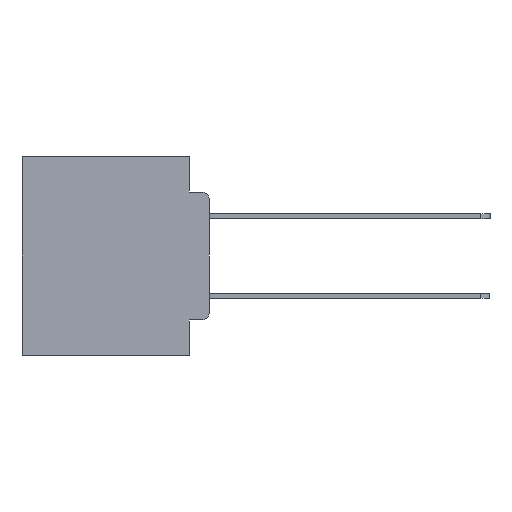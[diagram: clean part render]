
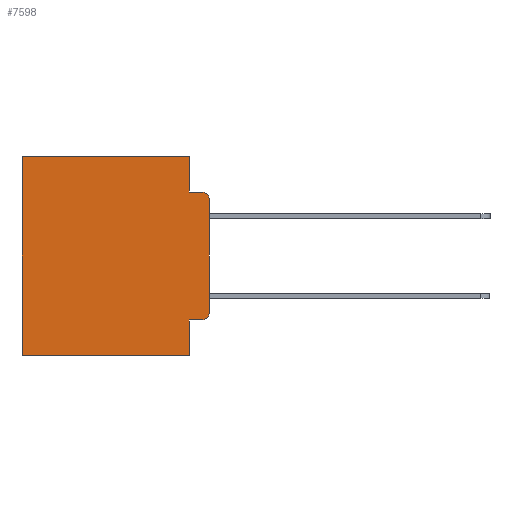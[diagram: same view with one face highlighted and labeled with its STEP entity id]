
A CAD part, left-side view. The second image highlights one B-rep face of the part: STEP entity #7598.
In plain terms, the highlighted planar face has unit normal (-1, 0, 0).
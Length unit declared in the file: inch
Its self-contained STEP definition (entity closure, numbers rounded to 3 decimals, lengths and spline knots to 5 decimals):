
#536 = EDGE_CURVE ( 'NONE', #15988, #26133, #26964, .T. ) ;
#649 = ORIENTED_EDGE ( 'NONE', *, *, #8804, .T. ) ;
#811 = VECTOR ( 'NONE', #26884, 39.37008 ) ;
#1095 = VECTOR ( 'NONE', #17243, 39.37008 ) ;
#1153 = FACE_OUTER_BOUND ( 'NONE', #25852, .T. ) ;
#1531 = CARTESIAN_POINT ( 'NONE',  ( 0.298, 0.473, 0. ) ) ;
#1646 = DIRECTION ( 'NONE',  ( -1., 0., 0. ) ) ;
#1666 = VECTOR ( 'NONE', #23406, 39.37008 ) ;
#1726 = CARTESIAN_POINT ( 'NONE',  ( 0.298, 0.051, -0.0885 ) ) ;
#2433 = EDGE_CURVE ( 'NONE', #15988, #26353, #12940, .T. ) ;
#2542 = ORIENTED_EDGE ( 'NONE', *, *, #2433, .F. ) ;
#2942 = CARTESIAN_POINT ( 'NONE',  ( 0.298, 0.051, -0.4115 ) ) ;
#4128 = CARTESIAN_POINT ( 'NONE',  ( 0.298, 0.02, -0.1085 ) ) ;
#4320 = ORIENTED_EDGE ( 'NONE', *, *, #12339, .F. ) ;
#4534 = ORIENTED_EDGE ( 'NONE', *, *, #19106, .T. ) ;
#4687 = VERTEX_POINT ( 'NONE', #25197 ) ;
#4892 = CARTESIAN_POINT ( 'NONE',  ( 0.298, 0.473, -0.5 ) ) ;
#4972 = ORIENTED_EDGE ( 'NONE', *, *, #25614, .F. ) ;
#5144 = DIRECTION ( 'NONE',  ( 0., -1., 0. ) ) ;
#5269 = AXIS2_PLACEMENT_3D ( 'NONE', #25804, #6248, #22928 ) ;
#5729 = ORIENTED_EDGE ( 'NONE', *, *, #23410, .F. ) ;
#5737 = ORIENTED_EDGE ( 'NONE', *, *, #19331, .T. ) ;
#6018 = AXIS2_PLACEMENT_3D ( 'NONE', #14471, #1646, #16541 ) ;
#6137 = LINE ( 'NONE', #11138, #1666 ) ;
#6248 = DIRECTION ( 'NONE',  ( 1., 0., 0. ) ) ;
#6474 = DIRECTION ( 'NONE',  ( 0., 1., 0. ) ) ;
#6486 = AXIS2_PLACEMENT_3D ( 'NONE', #4128, #9672, #23603 ) ;
#6606 = ORIENTED_EDGE ( 'NONE', *, *, #16039, .T. ) ;
#7159 = ORIENTED_EDGE ( 'NONE', *, *, #14793, .F. ) ;
#7250 = LINE ( 'NONE', #11858, #17108 ) ;
#7393 = LINE ( 'NONE', #1726, #12377 ) ;
#7552 = CARTESIAN_POINT ( 'NONE',  ( 0.298, 0.051, -0.0885 ) ) ;
#7598 = ADVANCED_FACE ( 'NONE', ( #1153 ), #25890, .F. ) ;
#8273 = DIRECTION ( 'NONE',  ( 0., -1., 0. ) ) ;
#8526 = CARTESIAN_POINT ( 'NONE',  ( 0.298, 0., -0.5 ) ) ;
#8598 = CIRCLE ( 'NONE', #6018, 0.02 ) ;
#8804 = EDGE_CURVE ( 'NONE', #4687, #13542, #11539, .T. ) ;
#9672 = DIRECTION ( 'NONE',  ( -1., 0., 0. ) ) ;
#11138 = CARTESIAN_POINT ( 'NONE',  ( 0.298, 0.051, 0. ) ) ;
#11351 = VERTEX_POINT ( 'NONE', #7552 ) ;
#11539 = LINE ( 'NONE', #2942, #21842 ) ;
#11803 = CARTESIAN_POINT ( 'NONE',  ( 0.298, 0.02, -0.0885 ) ) ;
#11858 = CARTESIAN_POINT ( 'NONE',  ( 0.298, 0.051, 0. ) ) ;
#12339 = EDGE_CURVE ( 'NONE', #4687, #13383, #6137, .T. ) ;
#12377 = VECTOR ( 'NONE', #8273, 39.37008 ) ;
#12391 = VERTEX_POINT ( 'NONE', #4892 ) ;
#12425 = VECTOR ( 'NONE', #16524, 39.37008 ) ;
#12910 = ORIENTED_EDGE ( 'NONE', *, *, #536, .T. ) ;
#12940 = LINE ( 'NONE', #13077, #811 ) ;
#13003 = CARTESIAN_POINT ( 'NONE',  ( 0.298, 0.02, -0.4115 ) ) ;
#13077 = CARTESIAN_POINT ( 'NONE',  ( 0.298, 0., 0. ) ) ;
#13383 = VERTEX_POINT ( 'NONE', #18697 ) ;
#13542 = VERTEX_POINT ( 'NONE', #13003 ) ;
#14471 = CARTESIAN_POINT ( 'NONE',  ( 0.298, 0.02, -0.3915 ) ) ;
#14793 = EDGE_CURVE ( 'NONE', #13383, #12391, #18486, .T. ) ;
#14939 = VERTEX_POINT ( 'NONE', #19170 ) ;
#15183 = CARTESIAN_POINT ( 'NONE',  ( 0.298, 0., 0. ) ) ;
#15988 = VERTEX_POINT ( 'NONE', #22478 ) ;
#16039 = EDGE_CURVE ( 'NONE', #22269, #12391, #23931, .T. ) ;
#16092 = DIRECTION ( 'NONE',  ( 0., 0., -1. ) ) ;
#16524 = DIRECTION ( 'NONE',  ( 0., 0., -1. ) ) ;
#16541 = DIRECTION ( 'NONE',  ( 0., 0., -1. ) ) ;
#16724 = CARTESIAN_POINT ( 'NONE',  ( 0.298, 0., -0.3915 ) ) ;
#17108 = VECTOR ( 'NONE', #16092, 39.37008 ) ;
#17243 = DIRECTION ( 'NONE',  ( 0., 1., 0. ) ) ;
#18056 = LINE ( 'NONE', #15183, #1095 ) ;
#18486 = LINE ( 'NONE', #8526, #23201 ) ;
#18697 = CARTESIAN_POINT ( 'NONE',  ( 0.298, 0.051, -0.5 ) ) ;
#19106 = EDGE_CURVE ( 'NONE', #13542, #26353, #8598, .T. ) ;
#19170 = CARTESIAN_POINT ( 'NONE',  ( 0.298, 0.051, 0. ) ) ;
#19331 = EDGE_CURVE ( 'NONE', #14939, #22269, #18056, .T. ) ;
#19956 = CARTESIAN_POINT ( 'NONE',  ( 0.298, 0.473, 0. ) ) ;
#21842 = VECTOR ( 'NONE', #5144, 39.37008 ) ;
#22269 = VERTEX_POINT ( 'NONE', #19956 ) ;
#22478 = CARTESIAN_POINT ( 'NONE',  ( 0.298, 0., -0.1085 ) ) ;
#22928 = DIRECTION ( 'NONE',  ( 0., 0., -1. ) ) ;
#23201 = VECTOR ( 'NONE', #6474, 39.37008 ) ;
#23406 = DIRECTION ( 'NONE',  ( 0., 0., -1. ) ) ;
#23410 = EDGE_CURVE ( 'NONE', #11351, #26133, #7393, .T. ) ;
#23603 = DIRECTION ( 'NONE',  ( 0., 0., -1. ) ) ;
#23931 = LINE ( 'NONE', #1531, #12425 ) ;
#25197 = CARTESIAN_POINT ( 'NONE',  ( 0.298, 0.051, -0.4115 ) ) ;
#25614 = EDGE_CURVE ( 'NONE', #14939, #11351, #7250, .T. ) ;
#25804 = CARTESIAN_POINT ( 'NONE',  ( 0.298, 0., 0. ) ) ;
#25852 = EDGE_LOOP ( 'NONE', ( #2542, #12910, #5729, #4972, #5737, #6606, #7159, #4320, #649, #4534 ) ) ;
#25890 = PLANE ( 'NONE',  #5269 ) ;
#26133 = VERTEX_POINT ( 'NONE', #11803 ) ;
#26353 = VERTEX_POINT ( 'NONE', #16724 ) ;
#26884 = DIRECTION ( 'NONE',  ( 0., 0., -1. ) ) ;
#26964 = CIRCLE ( 'NONE', #6486, 0.02 ) ;
